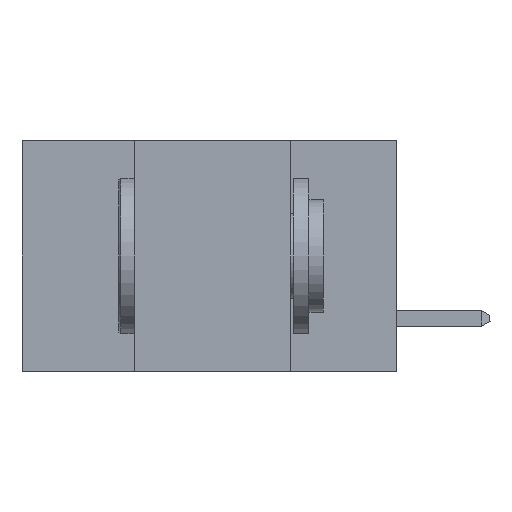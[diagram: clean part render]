
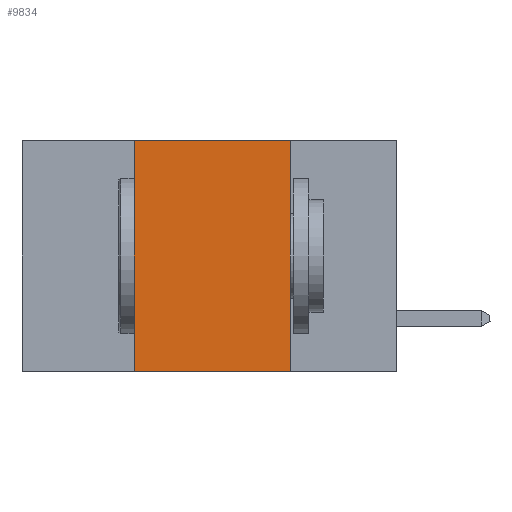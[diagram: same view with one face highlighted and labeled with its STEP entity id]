
A CAD part, left-side view. The second image highlights one B-rep face of the part: STEP entity #9834.
In plain terms, the highlighted planar face has unit normal (-1, 0, 0).
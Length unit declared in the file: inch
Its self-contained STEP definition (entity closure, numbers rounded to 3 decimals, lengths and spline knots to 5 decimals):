
#28 = LINE ( 'NONE', #17699, #4157 ) ;
#66 = VERTEX_POINT ( 'NONE', #5478 ) ;
#116 = VERTEX_POINT ( 'NONE', #1858 ) ;
#1044 = PLANE ( 'NONE',  #21400 ) ;
#1858 = CARTESIAN_POINT ( 'NONE',  ( 0., 0.42, 0. ) ) ;
#2379 = CARTESIAN_POINT ( 'NONE',  ( 0., 0.17, -0.37 ) ) ;
#3129 = DIRECTION ( 'NONE',  ( 0., -1., 0. ) ) ;
#3255 = LINE ( 'NONE', #15068, #12359 ) ;
#3602 = LINE ( 'NONE', #10984, #12732 ) ;
#4157 = VECTOR ( 'NONE', #19396, 39.37008 ) ;
#4273 = CARTESIAN_POINT ( 'NONE',  ( 0., 0.42, -0.37 ) ) ;
#5478 = CARTESIAN_POINT ( 'NONE',  ( 0., 0.17, 0. ) ) ;
#6617 = EDGE_CURVE ( 'NONE', #116, #66, #3602, .T. ) ;
#6786 = VECTOR ( 'NONE', #16338, 39.37008 ) ;
#7982 = CARTESIAN_POINT ( 'NONE',  ( 0., 0.6, 0. ) ) ;
#8575 = EDGE_CURVE ( 'NONE', #17651, #21111, #3255, .T. ) ;
#9735 = DIRECTION ( 'NONE',  ( 0., 0., -1. ) ) ;
#9834 = ADVANCED_FACE ( 'NONE', ( #16793 ), #1044, .F. ) ;
#10984 = CARTESIAN_POINT ( 'NONE',  ( 0., 0.6, 0. ) ) ;
#12166 = DIRECTION ( 'NONE',  ( 0., -1., 0. ) ) ;
#12359 = VECTOR ( 'NONE', #3129, 39.37008 ) ;
#12732 = VECTOR ( 'NONE', #12166, 39.37008 ) ;
#14638 = CARTESIAN_POINT ( 'NONE',  ( 0., 0.17, 0. ) ) ;
#15068 = CARTESIAN_POINT ( 'NONE',  ( 0., 0.6, -0.37 ) ) ;
#15392 = ORIENTED_EDGE ( 'NONE', *, *, #17689, .F. ) ;
#16338 = DIRECTION ( 'NONE',  ( 0., 0., -1. ) ) ;
#16579 = EDGE_CURVE ( 'NONE', #17651, #116, #28, .T. ) ;
#16793 = FACE_OUTER_BOUND ( 'NONE', #18324, .T. ) ;
#17651 = VERTEX_POINT ( 'NONE', #4273 ) ;
#17689 = EDGE_CURVE ( 'NONE', #66, #21111, #20351, .T. ) ;
#17699 = CARTESIAN_POINT ( 'NONE',  ( 0., 0.42, 0. ) ) ;
#18324 = EDGE_LOOP ( 'NONE', ( #15392, #20527, #18827, #18374 ) ) ;
#18374 = ORIENTED_EDGE ( 'NONE', *, *, #8575, .T. ) ;
#18827 = ORIENTED_EDGE ( 'NONE', *, *, #16579, .F. ) ;
#19396 = DIRECTION ( 'NONE',  ( 0., 0., 1. ) ) ;
#19886 = DIRECTION ( 'NONE',  ( 1., 0., 0. ) ) ;
#20351 = LINE ( 'NONE', #14638, #6786 ) ;
#20527 = ORIENTED_EDGE ( 'NONE', *, *, #6617, .F. ) ;
#21111 = VERTEX_POINT ( 'NONE', #2379 ) ;
#21400 = AXIS2_PLACEMENT_3D ( 'NONE', #7982, #19886, #9735 ) ;
